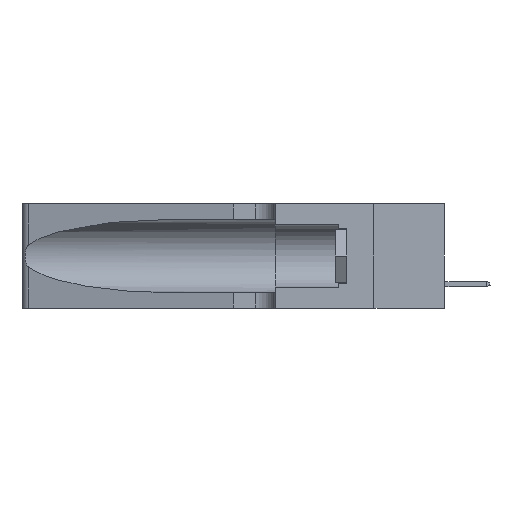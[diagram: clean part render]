
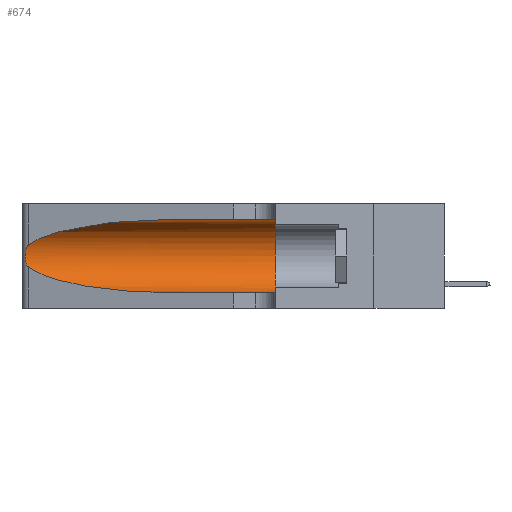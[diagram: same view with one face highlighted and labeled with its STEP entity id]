
A CAD part, left-side view. The second image highlights one B-rep face of the part: STEP entity #674.
In plain terms, the highlighted cylindrical face has radius 3.308 mm (diameter 6.617 mm), a partial arc.
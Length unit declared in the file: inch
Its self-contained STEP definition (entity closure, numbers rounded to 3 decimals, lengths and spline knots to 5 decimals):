
#674 = ADVANCED_FACE ( 'NONE', ( #12076 ), #4859, .F. ) ;
#1280 = ORIENTED_EDGE ( 'NONE', *, *, #6601, .F. ) ;
#1549 = CARTESIAN_POINT ( 'NONE',  ( 0.1305, 0.35, 0.31525 ) ) ;
#1648 = CARTESIAN_POINT ( 'NONE',  ( 0.1305, 0.35, 0.185 ) ) ;
#2566 = CARTESIAN_POINT ( 'NONE',  ( 0.26075, 1.23896, 0.178 ) ) ;
#2782 = CARTESIAN_POINT ( 'NONE',  ( 0.2373, 1.15595, 0.08982 ) ) ;
#2952 = B_SPLINE_CURVE_WITH_KNOTS ( 'NONE', 3,
 ( #17328, #6199, #13623, #6285, #4193, #4527, #4452, #2566, #8081, #13538, #19001, #9786, #20673, #4375 ),
 .UNSPECIFIED., .F., .F.,
 ( 4, 2, 2, 2, 2, 2, 4 ),
 ( 0., 0.00027, 0.00053, 0.00107, 0.0016, 0.00187, 0.00214 ),
 .UNSPECIFIED. ) ;
#2958 = EDGE_CURVE ( 'NONE', #17837, #20336, #23642, .T. ) ;
#3027 = CARTESIAN_POINT ( 'NONE',  ( 0.1305, 0.72297, 0.05475 ) ) ;
#4193 = CARTESIAN_POINT ( 'NONE',  ( 0.25854, 1.2359, 0.20912 ) ) ;
#4375 = CARTESIAN_POINT ( 'NONE',  ( 0.25487, 1.22718, 0.14631 ) ) ;
#4452 = CARTESIAN_POINT ( 'NONE',  ( 0.26075, 1.23896, 0.19203 ) ) ;
#4527 = CARTESIAN_POINT ( 'NONE',  ( 0.26018, 1.23835, 0.19895 ) ) ;
#4859 = CYLINDRICAL_SURFACE ( 'NONE', #19609, 0.13025 ) ;
#4909 = LINE ( 'NONE', #5437, #15267 ) ;
#4918 = EDGE_CURVE ( 'NONE', #17837, #11251, #22913, .T. ) ;
#5437 = CARTESIAN_POINT ( 'NONE',  ( 0.1305, 1.61858, 0.05475 ) ) ;
#6199 = CARTESIAN_POINT ( 'NONE',  ( 0.25555, 1.22994, 0.2215 ) ) ;
#6285 = CARTESIAN_POINT ( 'NONE',  ( 0.25787, 1.23484, 0.2124 ) ) ;
#6510 =( BOUNDED_CURVE ( )  B_SPLINE_CURVE ( 3, ( #10405, #2782, #14062, #3027 ),
 .UNSPECIFIED., .F., .F. ) 
 B_SPLINE_CURVE_WITH_KNOTS ( ( 4, 4 ),
 ( 3.44316, 4.71239 ),
 .UNSPECIFIED. ) 
 CURVE ( )  GEOMETRIC_REPRESENTATION_ITEM ( )  RATIONAL_B_SPLINE_CURVE ( ( 1., 0.87, 0.87, 1. ) ) 
 REPRESENTATION_ITEM ( '' )  );
#6601 = EDGE_CURVE ( 'NONE', #20336, #13126, #16253, .T. ) ;
#6843 = VERTEX_POINT ( 'NONE', #17887 ) ;
#7013 = CARTESIAN_POINT ( 'NONE',  ( 0.25487, 1.22718, 0.22369 ) ) ;
#8007 = AXIS2_PLACEMENT_3D ( 'NONE', #1648, #23716, #12666 ) ;
#8014 = CARTESIAN_POINT ( 'NONE',  ( 0.1305, 0.35, 0.05475 ) ) ;
#8081 = CARTESIAN_POINT ( 'NONE',  ( 0.26017, 1.23833, 0.17102 ) ) ;
#9249 = DIRECTION ( 'NONE',  ( 0., -1., 0. ) ) ;
#9786 = CARTESIAN_POINT ( 'NONE',  ( 0.25639, 1.23186, 0.15144 ) ) ;
#10405 = CARTESIAN_POINT ( 'NONE',  ( 0.25487, 1.22718, 0.14631 ) ) ;
#10752 = ORIENTED_EDGE ( 'NONE', *, *, #2958, .F. ) ;
#11112 = VERTEX_POINT ( 'NONE', #18992 ) ;
#11177 = CARTESIAN_POINT ( 'NONE',  ( 0.2373, 1.15595, 0.28018 ) ) ;
#11251 = VERTEX_POINT ( 'NONE', #7013 ) ;
#12076 = FACE_OUTER_BOUND ( 'NONE', #23885, .T. ) ;
#12517 = CARTESIAN_POINT ( 'NONE',  ( 0.1305, 1.61858, 0.31525 ) ) ;
#12666 = DIRECTION ( 'NONE',  ( 0., 0., 1. ) ) ;
#12919 = CARTESIAN_POINT ( 'NONE',  ( 0.1305, 0.72297, 0.31525 ) ) ;
#13126 = VERTEX_POINT ( 'NONE', #8014 ) ;
#13538 = CARTESIAN_POINT ( 'NONE',  ( 0.25856, 1.23593, 0.16098 ) ) ;
#13623 = CARTESIAN_POINT ( 'NONE',  ( 0.25639, 1.23184, 0.21858 ) ) ;
#13788 = ORIENTED_EDGE ( 'NONE', *, *, #14309, .T. ) ;
#14062 = CARTESIAN_POINT ( 'NONE',  ( 0.18966, 0.96281, 0.05475 ) ) ;
#14309 = EDGE_CURVE ( 'NONE', #6843, #13126, #4909, .T. ) ;
#14653 = DIRECTION ( 'NONE',  ( 0., -1., 0. ) ) ;
#14696 = CARTESIAN_POINT ( 'NONE',  ( 0.25487, 1.22718, 0.22369 ) ) ;
#15154 = ORIENTED_EDGE ( 'NONE', *, *, #16384, .T. ) ;
#15267 = VECTOR ( 'NONE', #9249, 39.37008 ) ;
#16113 = DIRECTION ( 'NONE',  ( 0., 0., -1. ) ) ;
#16253 = CIRCLE ( 'NONE', #8007, 0.13025 ) ;
#16384 = EDGE_CURVE ( 'NONE', #11251, #11112, #2952, .T. ) ;
#16579 = ORIENTED_EDGE ( 'NONE', *, *, #4918, .T. ) ;
#17328 = CARTESIAN_POINT ( 'NONE',  ( 0.25487, 1.22718, 0.22369 ) ) ;
#17837 = VERTEX_POINT ( 'NONE', #18740 ) ;
#17858 = VECTOR ( 'NONE', #21894, 39.37008 ) ;
#17887 = CARTESIAN_POINT ( 'NONE',  ( 0.1305, 0.72297, 0.05475 ) ) ;
#18035 = CARTESIAN_POINT ( 'NONE',  ( 0.1305, 1.61858, 0.185 ) ) ;
#18740 = CARTESIAN_POINT ( 'NONE',  ( 0.1305, 0.72297, 0.31525 ) ) ;
#18992 = CARTESIAN_POINT ( 'NONE',  ( 0.25487, 1.22718, 0.14631 ) ) ;
#19001 = CARTESIAN_POINT ( 'NONE',  ( 0.25789, 1.23486, 0.15765 ) ) ;
#19609 = AXIS2_PLACEMENT_3D ( 'NONE', #18035, #14653, #16113 ) ;
#19977 = CARTESIAN_POINT ( 'NONE',  ( 0.18966, 0.96281, 0.31525 ) ) ;
#20336 = VERTEX_POINT ( 'NONE', #1549 ) ;
#20673 = CARTESIAN_POINT ( 'NONE',  ( 0.25555, 1.22993, 0.14849 ) ) ;
#21059 = ORIENTED_EDGE ( 'NONE', *, *, #22839, .T. ) ;
#21894 = DIRECTION ( 'NONE',  ( 0., -1., 0. ) ) ;
#22839 = EDGE_CURVE ( 'NONE', #11112, #6843, #6510, .T. ) ;
#22913 =( BOUNDED_CURVE ( )  B_SPLINE_CURVE ( 3, ( #12919, #19977, #11177, #14696 ),
 .UNSPECIFIED., .F., .F. ) 
 B_SPLINE_CURVE_WITH_KNOTS ( ( 4, 4 ),
 ( 1.5708, 2.84003 ),
 .UNSPECIFIED. ) 
 CURVE ( )  GEOMETRIC_REPRESENTATION_ITEM ( )  RATIONAL_B_SPLINE_CURVE ( ( 1., 0.87, 0.87, 1. ) ) 
 REPRESENTATION_ITEM ( '' )  );
#23642 = LINE ( 'NONE', #12517, #17858 ) ;
#23716 = DIRECTION ( 'NONE',  ( 0., 1., 0. ) ) ;
#23885 = EDGE_LOOP ( 'NONE', ( #16579, #15154, #21059, #13788, #1280, #10752 ) ) ;
